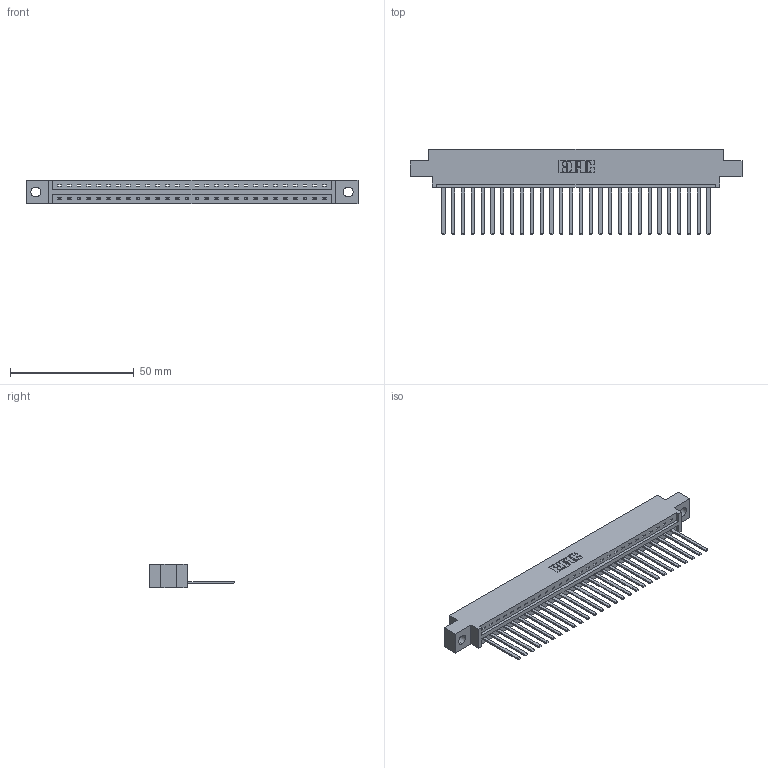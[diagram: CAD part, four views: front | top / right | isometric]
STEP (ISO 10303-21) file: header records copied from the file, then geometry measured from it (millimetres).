
FILE_DESCRIPTION (( 'STEP AP203' ), '1' );
FILE_NAME ('337-028-544-604.STEP', '2018-08-06T11:28:17', ( '' ), ( '' ), 'SwSTEP 2.0', 'SolidWorks 2016', '' );
FILE_SCHEMA (( 'CONFIG_CONTROL_DESIGN' ));
Length unit declared in the file: inch
Products named in the file (3): 337 Part_0.170 Offset - 0.156 Dia-TH; 345-292-001_345-293-144; 337-028-544-604
Assembly tree (29 placements, depth 2):
  337-028-544-604
    337 Part_0.170 Offset - 0.156 Dia-TH
    345-292-001_345-293-144  x28
Bounding box: 133.96 x 34.3 x 9.4 mm (x, y, z)
Volume: 13866.6 mm3; surface area: 15209.8 mm2
Topology: 29 solids, 29 shells, 1686 faces, 5083 edges, 3350 vertices
Faces by surface type: plane 1250, cylinder 436
Entity records: 22575 total; most frequent: CARTESIAN_POINT 3938, ORIENTED_EDGE 3902, DIRECTION 3339, EDGE_CURVE 1951, VECTOR 1827, LINE 1827, VERTEX_POINT 1298, AXIS2_PLACEMENT_3D 756
